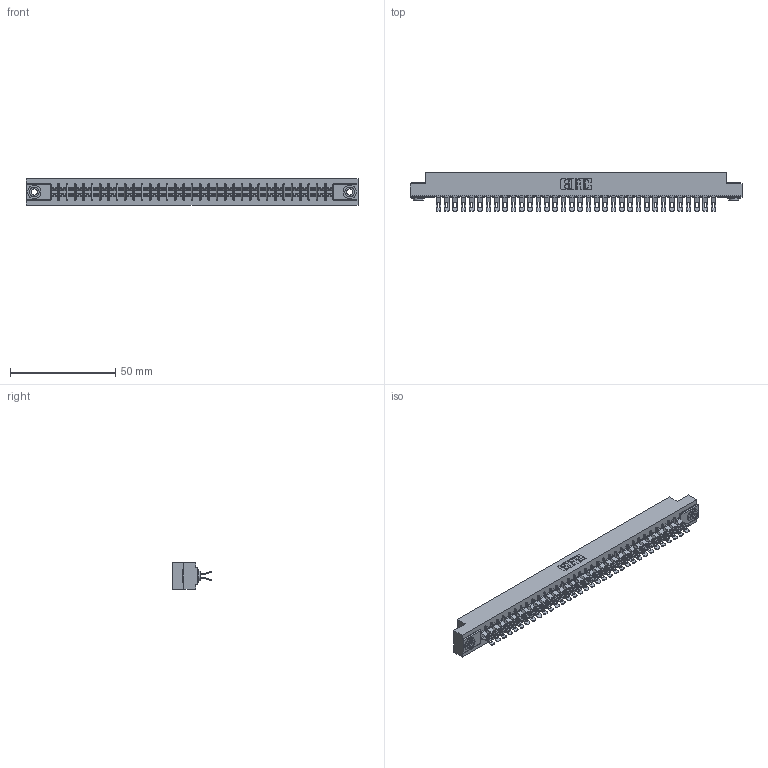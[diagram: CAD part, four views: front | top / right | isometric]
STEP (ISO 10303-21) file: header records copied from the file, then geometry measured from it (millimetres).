
FILE_DESCRIPTION (( 'STEP AP203' ), '1' );
FILE_NAME ('355-068-555-503.STEP', '2019-09-12T17:06:13', ( '' ), ( '' ), 'SwSTEP 2.0', 'SolidWorks 2016', '' );
FILE_SCHEMA (( 'CONFIG_CONTROL_DESIGN' ));
Length unit declared in the file: inch
Products named in the file (4): 305-290-001_555; 355-068-555-503; 305 Part_.156 Dia; 345-250-002_345-250-002-102
Assembly tree (71 placements, depth 2):
  355-068-555-503
    305 Part_.156 Dia
    305-290-001_555  x68
    345-250-002_345-250-002-102  x2
Bounding box: 157.73 x 18.41 x 12.7 mm (x, y, z)
Volume: 16139 mm3; surface area: 22634.1 mm2
Topology: 71 solids, 71 shells, 4656 faces, 13858 edges, 9052 vertices
Faces by surface type: plane 2268, cylinder 2244, sphere 136, cone 8
Entity records: 39476 total; most frequent: CARTESIAN_POINT 6531, ORIENTED_EDGE 6464, DIRECTION 6334, EDGE_CURVE 3232, LINE 2576, VECTOR 2576, VERTEX_POINT 2060, AXIS2_PLACEMENT_3D 1879
